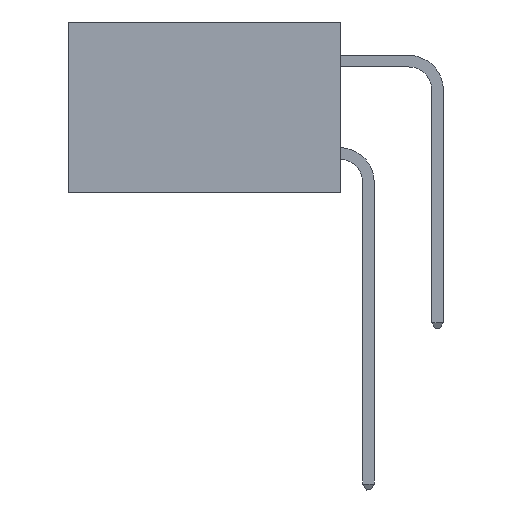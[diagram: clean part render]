
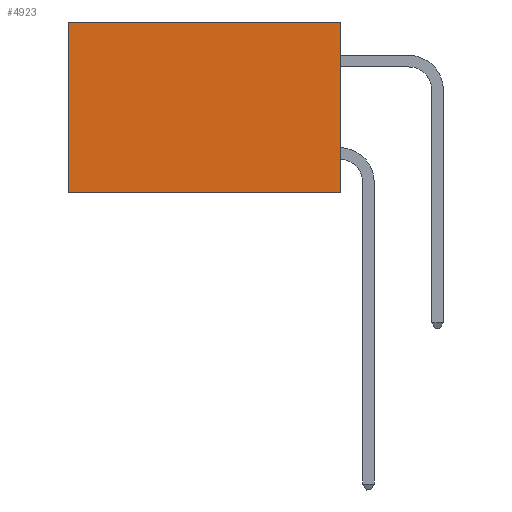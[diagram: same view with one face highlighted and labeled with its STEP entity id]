
A CAD part, left-side view. The second image highlights one B-rep face of the part: STEP entity #4923.
In plain terms, the highlighted planar face has unit normal (-1, 0, 0).
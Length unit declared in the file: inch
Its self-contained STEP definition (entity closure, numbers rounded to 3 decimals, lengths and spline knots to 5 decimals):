
#214 = LINE ( 'NONE', #24119, #17238 ) ;
#1250 = VECTOR ( 'NONE', #3442, 39.37008 ) ;
#1360 = PLANE ( 'NONE',  #14725 ) ;
#1609 = CARTESIAN_POINT ( 'NONE',  ( 0.277, 0.59, -0.37 ) ) ;
#2201 = ORIENTED_EDGE ( 'NONE', *, *, #2521, .F. ) ;
#2521 = EDGE_CURVE ( 'NONE', #4694, #5699, #214, .T. ) ;
#3442 = DIRECTION ( 'NONE',  ( 0., 1., 0. ) ) ;
#3622 = CARTESIAN_POINT ( 'NONE',  ( 0.277, 0., 0. ) ) ;
#4694 = VERTEX_POINT ( 'NONE', #3622 ) ;
#4923 = ADVANCED_FACE ( 'NONE', ( #26968 ), #1360, .F. ) ;
#5699 = VERTEX_POINT ( 'NONE', #27654 ) ;
#5916 = CARTESIAN_POINT ( 'NONE',  ( 0.277, 0., -0.37 ) ) ;
#6479 = EDGE_CURVE ( 'NONE', #27054, #18785, #27648, .T. ) ;
#7721 = DIRECTION ( 'NONE',  ( 0., 0., -1. ) ) ;
#7785 = DIRECTION ( 'NONE',  ( 1., 0., 0. ) ) ;
#7885 = CARTESIAN_POINT ( 'NONE',  ( 0.277, 0., -0.37 ) ) ;
#10914 = EDGE_CURVE ( 'NONE', #5699, #18785, #17923, .T. ) ;
#11378 = VECTOR ( 'NONE', #12585, 39.37008 ) ;
#12585 = DIRECTION ( 'NONE',  ( 0., 1., 0. ) ) ;
#14609 = EDGE_LOOP ( 'NONE', ( #16670, #16422, #2201, #22260 ) ) ;
#14725 = AXIS2_PLACEMENT_3D ( 'NONE', #7885, #7785, #7721 ) ;
#15658 = EDGE_CURVE ( 'NONE', #4694, #27054, #18220, .T. ) ;
#16422 = ORIENTED_EDGE ( 'NONE', *, *, #10914, .F. ) ;
#16670 = ORIENTED_EDGE ( 'NONE', *, *, #6479, .T. ) ;
#16702 = CARTESIAN_POINT ( 'NONE',  ( 0.277, 0., 0. ) ) ;
#17238 = VECTOR ( 'NONE', #24084, 39.37008 ) ;
#17923 = LINE ( 'NONE', #5916, #11378 ) ;
#18220 = LINE ( 'NONE', #16702, #1250 ) ;
#18785 = VERTEX_POINT ( 'NONE', #1609 ) ;
#21215 = VECTOR ( 'NONE', #25211, 39.37008 ) ;
#22260 = ORIENTED_EDGE ( 'NONE', *, *, #15658, .T. ) ;
#22523 = CARTESIAN_POINT ( 'NONE',  ( 0.277, 0.59, 0. ) ) ;
#24084 = DIRECTION ( 'NONE',  ( 0., 0., -1. ) ) ;
#24119 = CARTESIAN_POINT ( 'NONE',  ( 0.277, 0., -0.37 ) ) ;
#25211 = DIRECTION ( 'NONE',  ( 0., 0., -1. ) ) ;
#26968 = FACE_OUTER_BOUND ( 'NONE', #14609, .T. ) ;
#27054 = VERTEX_POINT ( 'NONE', #22523 ) ;
#27648 = LINE ( 'NONE', #27799, #21215 ) ;
#27654 = CARTESIAN_POINT ( 'NONE',  ( 0.277, 0., -0.37 ) ) ;
#27799 = CARTESIAN_POINT ( 'NONE',  ( 0.277, 0.59, -0.37 ) ) ;
